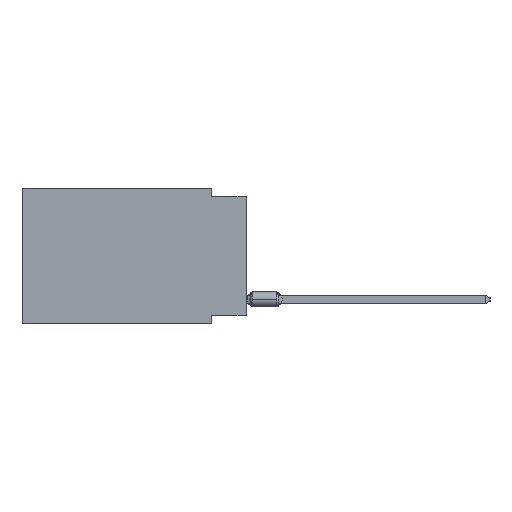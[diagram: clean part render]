
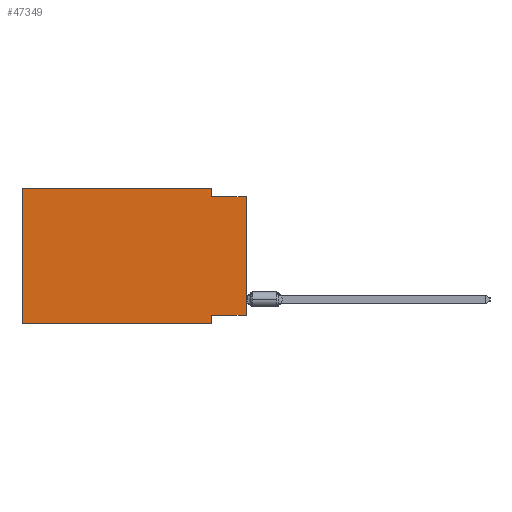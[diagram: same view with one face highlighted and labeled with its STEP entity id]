
A CAD part, left-side view. The second image highlights one B-rep face of the part: STEP entity #47349.
In plain terms, the highlighted planar face has unit normal (-1, 0, 0).
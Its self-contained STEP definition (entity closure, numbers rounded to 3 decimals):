
#783 = EDGE_CURVE ( 'NONE', #53532, #37814, #49040, .T. ) ;
#1273 = LINE ( 'NONE', #37800, #12106 ) ;
#3520 = VERTEX_POINT ( 'NONE', #22564 ) ;
#4287 = CARTESIAN_POINT ( 'NONE',  ( 0., 16.383, -9.906 ) ) ;
#5247 = DIRECTION ( 'NONE',  ( 0., 0., -1. ) ) ;
#6429 = DIRECTION ( 'NONE',  ( 1., 0., 0. ) ) ;
#6930 = VECTOR ( 'NONE', #5247, 1000. ) ;
#7428 = VECTOR ( 'NONE', #16907, 1000. ) ;
#7912 = VERTEX_POINT ( 'NONE', #26586 ) ;
#9556 = LINE ( 'NONE', #16945, #39003 ) ;
#10261 = ORIENTED_EDGE ( 'NONE', *, *, #39442, .F. ) ;
#11500 = DIRECTION ( 'NONE',  ( 0., -1., 0. ) ) ;
#11729 = CARTESIAN_POINT ( 'NONE',  ( 0., 0., -9.271 ) ) ;
#12106 = VECTOR ( 'NONE', #34263, 1000. ) ;
#12573 = CARTESIAN_POINT ( 'NONE',  ( 0., 2.54, -0.635 ) ) ;
#15809 = EDGE_CURVE ( 'NONE', #3520, #39685, #48095, .T. ) ;
#15976 = ORIENTED_EDGE ( 'NONE', *, *, #21119, .F. ) ;
#16907 = DIRECTION ( 'NONE',  ( 0., 1., 0. ) ) ;
#16945 = CARTESIAN_POINT ( 'NONE',  ( 0., 16.383, -9.906 ) ) ;
#17665 = FACE_OUTER_BOUND ( 'NONE', #43103, .T. ) ;
#20907 = EDGE_CURVE ( 'NONE', #37814, #21123, #46127, .T. ) ;
#21119 = EDGE_CURVE ( 'NONE', #39685, #28125, #31685, .T. ) ;
#21123 = VERTEX_POINT ( 'NONE', #44198 ) ;
#22564 = CARTESIAN_POINT ( 'NONE',  ( 0., 2.54, 0. ) ) ;
#22995 = VECTOR ( 'NONE', #51620, 1000. ) ;
#23356 = VERTEX_POINT ( 'NONE', #4287 ) ;
#25149 = VECTOR ( 'NONE', #52453, 1000. ) ;
#26002 = CARTESIAN_POINT ( 'NONE',  ( 0., 2.54, -9.906 ) ) ;
#26051 = ORIENTED_EDGE ( 'NONE', *, *, #783, .F. ) ;
#26586 = CARTESIAN_POINT ( 'NONE',  ( 0., 16.383, 0. ) ) ;
#28125 = VERTEX_POINT ( 'NONE', #39024 ) ;
#29243 = EDGE_CURVE ( 'NONE', #53532, #28125, #1273, .T. ) ;
#31400 = VECTOR ( 'NONE', #11500, 1000. ) ;
#31685 = LINE ( 'NONE', #49079, #31400 ) ;
#33559 = DIRECTION ( 'NONE',  ( 0., -1., 0. ) ) ;
#34263 = DIRECTION ( 'NONE',  ( 0., 0., 1. ) ) ;
#35515 = LINE ( 'NONE', #43133, #40974 ) ;
#37800 = CARTESIAN_POINT ( 'NONE',  ( 0., 0., 0. ) ) ;
#37814 = VERTEX_POINT ( 'NONE', #49360 ) ;
#38081 = PLANE ( 'NONE',  #51943 ) ;
#39003 = VECTOR ( 'NONE', #33559, 1000. ) ;
#39024 = CARTESIAN_POINT ( 'NONE',  ( 0., 0., -0.635 ) ) ;
#39442 = EDGE_CURVE ( 'NONE', #7912, #3520, #35515, .T. ) ;
#39685 = VERTEX_POINT ( 'NONE', #12573 ) ;
#39957 = DIRECTION ( 'NONE',  ( 0., 0., -1. ) ) ;
#40193 = CARTESIAN_POINT ( 'NONE',  ( 0., 2.54, 0. ) ) ;
#40627 = ORIENTED_EDGE ( 'NONE', *, *, #20907, .F. ) ;
#40974 = VECTOR ( 'NONE', #51277, 1000. ) ;
#41829 = LINE ( 'NONE', #52153, #22995 ) ;
#43103 = EDGE_LOOP ( 'NONE', ( #52007, #15976, #45645, #10261, #46365, #43577, #40627, #26051 ) ) ;
#43133 = CARTESIAN_POINT ( 'NONE',  ( 0., 16.383, 0. ) ) ;
#43201 = CARTESIAN_POINT ( 'NONE',  ( 0., 0., -9.271 ) ) ;
#43557 = EDGE_CURVE ( 'NONE', #23356, #21123, #9556, .T. ) ;
#43577 = ORIENTED_EDGE ( 'NONE', *, *, #43557, .T. ) ;
#44198 = CARTESIAN_POINT ( 'NONE',  ( 0., 2.54, -9.906 ) ) ;
#45645 = ORIENTED_EDGE ( 'NONE', *, *, #15809, .F. ) ;
#46127 = LINE ( 'NONE', #26002, #6930 ) ;
#46365 = ORIENTED_EDGE ( 'NONE', *, *, #51103, .F. ) ;
#47349 = ADVANCED_FACE ( 'NONE', ( #17665 ), #38081, .F. ) ;
#48095 = LINE ( 'NONE', #40193, #25149 ) ;
#49040 = LINE ( 'NONE', #11729, #7428 ) ;
#49079 = CARTESIAN_POINT ( 'NONE',  ( 0., 0., -0.635 ) ) ;
#49360 = CARTESIAN_POINT ( 'NONE',  ( 0., 2.54, -9.271 ) ) ;
#50590 = CARTESIAN_POINT ( 'NONE',  ( 0., 16.383, 0. ) ) ;
#51103 = EDGE_CURVE ( 'NONE', #23356, #7912, #41829, .T. ) ;
#51277 = DIRECTION ( 'NONE',  ( 0., -1., 0. ) ) ;
#51620 = DIRECTION ( 'NONE',  ( 0., 0., 1. ) ) ;
#51943 = AXIS2_PLACEMENT_3D ( 'NONE', #50590, #6429, #39957 ) ;
#52007 = ORIENTED_EDGE ( 'NONE', *, *, #29243, .T. ) ;
#52153 = CARTESIAN_POINT ( 'NONE',  ( 0., 16.383, 0. ) ) ;
#52453 = DIRECTION ( 'NONE',  ( 0., 0., -1. ) ) ;
#53532 = VERTEX_POINT ( 'NONE', #43201 ) ;
